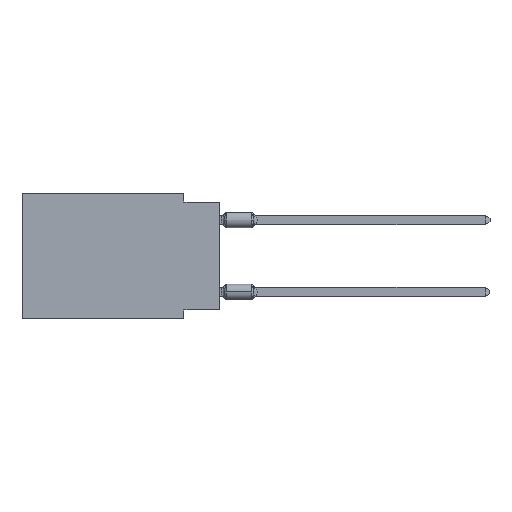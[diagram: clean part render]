
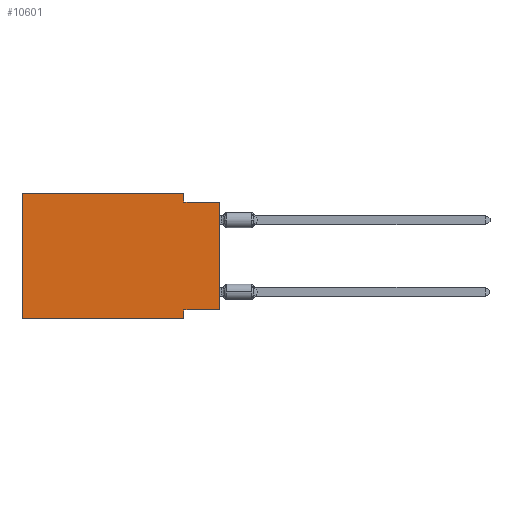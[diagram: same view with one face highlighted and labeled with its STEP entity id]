
A CAD part, left-side view. The second image highlights one B-rep face of the part: STEP entity #10601.
In plain terms, the highlighted planar face has unit normal (-1, 0, 0).
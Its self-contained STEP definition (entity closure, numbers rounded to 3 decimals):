
#91 = LINE ( 'NONE', #6665, #16577 ) ;
#611 = CARTESIAN_POINT ( 'NONE',  ( 0., 0., -0.635 ) ) ;
#1601 = VERTEX_POINT ( 'NONE', #4511 ) ;
#2103 = ORIENTED_EDGE ( 'NONE', *, *, #21156, .F. ) ;
#2402 = EDGE_CURVE ( 'NONE', #15863, #15378, #10991, .T. ) ;
#2537 = ORIENTED_EDGE ( 'NONE', *, *, #20544, .F. ) ;
#2854 = DIRECTION ( 'NONE',  ( 0., 0., -1. ) ) ;
#3043 = CARTESIAN_POINT ( 'NONE',  ( 0., 13.97, 0. ) ) ;
#3377 = VERTEX_POINT ( 'NONE', #611 ) ;
#3727 = EDGE_CURVE ( 'NONE', #11322, #3377, #13772, .T. ) ;
#3774 = VECTOR ( 'NONE', #2854, 1000. ) ;
#4405 = PLANE ( 'NONE',  #9599 ) ;
#4469 = CARTESIAN_POINT ( 'NONE',  ( 0., 2.54, 0. ) ) ;
#4511 = CARTESIAN_POINT ( 'NONE',  ( 0., 13.97, -8.89 ) ) ;
#6211 = ORIENTED_EDGE ( 'NONE', *, *, #2402, .F. ) ;
#6665 = CARTESIAN_POINT ( 'NONE',  ( 0., 0., -0.635 ) ) ;
#6708 = CARTESIAN_POINT ( 'NONE',  ( 0., 2.54, -8.89 ) ) ;
#6709 = ORIENTED_EDGE ( 'NONE', *, *, #3727, .T. ) ;
#6767 = VECTOR ( 'NONE', #16422, 1000. ) ;
#6980 = CARTESIAN_POINT ( 'NONE',  ( 0., 2.54, 0. ) ) ;
#7361 = CARTESIAN_POINT ( 'NONE',  ( 0., 0., -8.255 ) ) ;
#8065 = CARTESIAN_POINT ( 'NONE',  ( 0., 2.54, -0.635 ) ) ;
#8094 = ORIENTED_EDGE ( 'NONE', *, *, #13116, .F. ) ;
#8962 = VERTEX_POINT ( 'NONE', #13885 ) ;
#9248 = DIRECTION ( 'NONE',  ( 0., 0., -1. ) ) ;
#9346 = FACE_OUTER_BOUND ( 'NONE', #13957, .T. ) ;
#9360 = CARTESIAN_POINT ( 'NONE',  ( 0., 13.97, 0. ) ) ;
#9452 = CARTESIAN_POINT ( 'NONE',  ( 0., 13.97, -8.89 ) ) ;
#9566 = DIRECTION ( 'NONE',  ( 0., -1., 0. ) ) ;
#9599 = AXIS2_PLACEMENT_3D ( 'NONE', #11060, #18852, #9248 ) ;
#10287 = VECTOR ( 'NONE', #9566, 1000. ) ;
#10601 = ADVANCED_FACE ( 'NONE', ( #9346 ), #4405, .F. ) ;
#10794 = VECTOR ( 'NONE', #17932, 1000. ) ;
#10881 = DIRECTION ( 'NONE',  ( 0., -1., 0. ) ) ;
#10991 = LINE ( 'NONE', #3043, #11850 ) ;
#11060 = CARTESIAN_POINT ( 'NONE',  ( 0., 13.97, 0. ) ) ;
#11121 = VERTEX_POINT ( 'NONE', #15521 ) ;
#11322 = VERTEX_POINT ( 'NONE', #7361 ) ;
#11850 = VECTOR ( 'NONE', #10881, 1000. ) ;
#12726 = CARTESIAN_POINT ( 'NONE',  ( 0., 0., -8.255 ) ) ;
#13020 = ORIENTED_EDGE ( 'NONE', *, *, #17849, .F. ) ;
#13116 = EDGE_CURVE ( 'NONE', #8962, #11121, #14718, .T. ) ;
#13386 = VECTOR ( 'NONE', #14052, 1000. ) ;
#13772 = LINE ( 'NONE', #15235, #15642 ) ;
#13828 = ORIENTED_EDGE ( 'NONE', *, *, #18899, .F. ) ;
#13840 = LINE ( 'NONE', #20343, #13386 ) ;
#13885 = CARTESIAN_POINT ( 'NONE',  ( 0., 2.54, -8.255 ) ) ;
#13957 = EDGE_LOOP ( 'NONE', ( #6709, #13828, #2103, #6211, #2537, #16137, #8094, #13020 ) ) ;
#14052 = DIRECTION ( 'NONE',  ( 0., 0., 1. ) ) ;
#14477 = LINE ( 'NONE', #9452, #10287 ) ;
#14519 = LINE ( 'NONE', #12726, #10794 ) ;
#14718 = LINE ( 'NONE', #6708, #6767 ) ;
#15235 = CARTESIAN_POINT ( 'NONE',  ( 0., 0., 0. ) ) ;
#15240 = VERTEX_POINT ( 'NONE', #8065 ) ;
#15378 = VERTEX_POINT ( 'NONE', #6980 ) ;
#15521 = CARTESIAN_POINT ( 'NONE',  ( 0., 2.54, -8.89 ) ) ;
#15642 = VECTOR ( 'NONE', #20371, 1000. ) ;
#15863 = VERTEX_POINT ( 'NONE', #9360 ) ;
#16137 = ORIENTED_EDGE ( 'NONE', *, *, #19787, .T. ) ;
#16422 = DIRECTION ( 'NONE',  ( 0., 0., -1. ) ) ;
#16577 = VECTOR ( 'NONE', #19702, 1000. ) ;
#17849 = EDGE_CURVE ( 'NONE', #11322, #8962, #14519, .T. ) ;
#17932 = DIRECTION ( 'NONE',  ( 0., 1., 0. ) ) ;
#18852 = DIRECTION ( 'NONE',  ( 1., 0., 0. ) ) ;
#18899 = EDGE_CURVE ( 'NONE', #15240, #3377, #91, .T. ) ;
#19702 = DIRECTION ( 'NONE',  ( 0., -1., 0. ) ) ;
#19787 = EDGE_CURVE ( 'NONE', #1601, #11121, #14477, .T. ) ;
#20343 = CARTESIAN_POINT ( 'NONE',  ( 0., 13.97, 0. ) ) ;
#20371 = DIRECTION ( 'NONE',  ( 0., 0., 1. ) ) ;
#20544 = EDGE_CURVE ( 'NONE', #1601, #15863, #13840, .T. ) ;
#21156 = EDGE_CURVE ( 'NONE', #15378, #15240, #21174, .T. ) ;
#21174 = LINE ( 'NONE', #4469, #3774 ) ;
